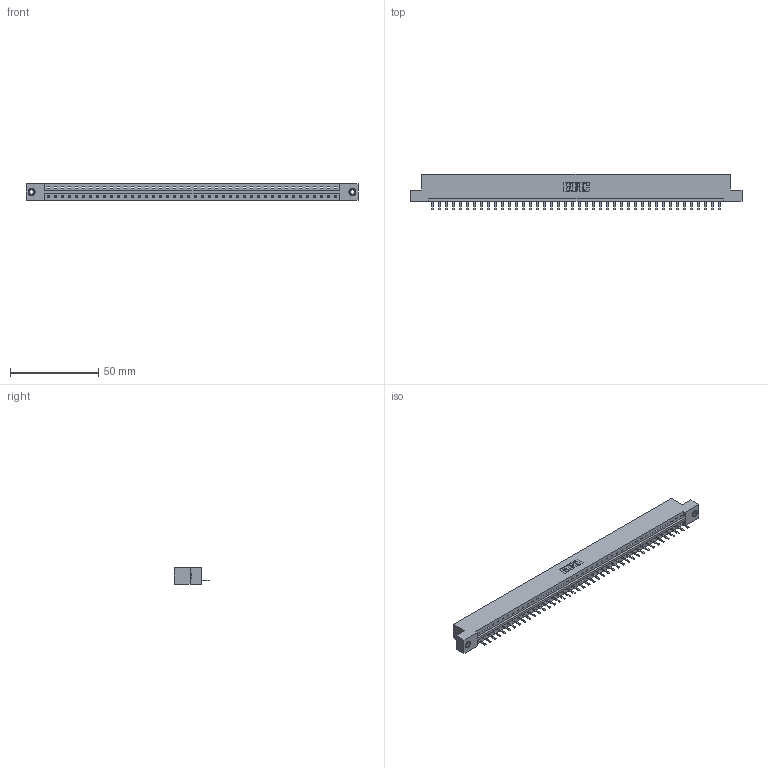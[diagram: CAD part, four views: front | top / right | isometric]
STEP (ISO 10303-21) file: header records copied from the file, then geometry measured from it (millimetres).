
FILE_DESCRIPTION (( 'STEP AP203' ), '1' );
FILE_NAME ('333-042-520-107.STEP', '2018-08-03T16:03:54', ( '' ), ( '' ), 'SwSTEP 2.0', 'SolidWorks 2016', '' );
FILE_SCHEMA (( 'CONFIG_CONTROL_DESIGN' ));
Length unit declared in the file: inch
Products named in the file (4): 345-250-001_345-250-005-103; 333-042-520-107; 333 Part_Flush - .156 Dia - TI; 345-292-001_345-293-120
Assembly tree (45 placements, depth 2):
  333-042-520-107
    333 Part_Flush - .156 Dia - TI
    345-292-001_345-293-120  x42
    345-250-001_345-250-005-103  x2
Bounding box: 187.96 x 20.02 x 9.4 mm (x, y, z)
Volume: 18779.7 mm3; surface area: 19933.1 mm2
Topology: 45 solids, 45 shells, 2778 faces, 8175 edges, 5330 vertices
Faces by surface type: plane 1950, cylinder 812, cone 12, torus 4
Entity records: 26976 total; most frequent: CARTESIAN_POINT 4647, ORIENTED_EDGE 4606, DIRECTION 3941, EDGE_CURVE 2303, LINE 2151, VECTOR 2151, VERTEX_POINT 1528, AXIS2_PLACEMENT_3D 895
